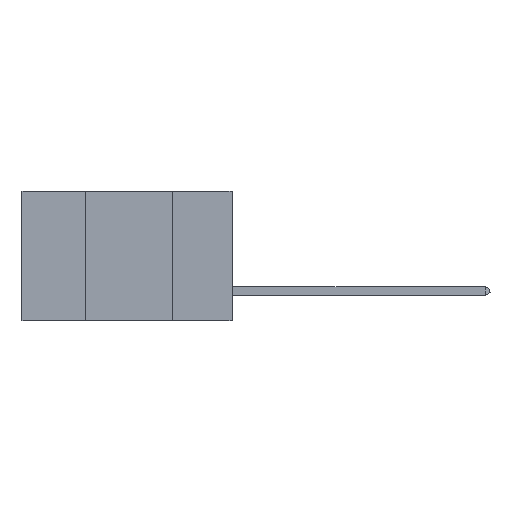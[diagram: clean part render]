
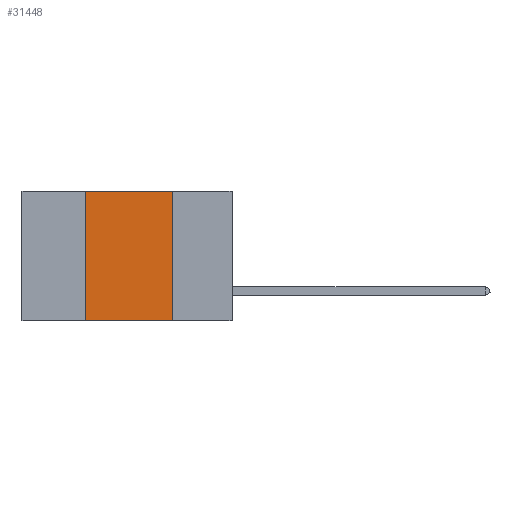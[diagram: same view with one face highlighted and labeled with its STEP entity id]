
A CAD part, left-side view. The second image highlights one B-rep face of the part: STEP entity #31448.
In plain terms, the highlighted planar face has unit normal (-1, 0, 0).
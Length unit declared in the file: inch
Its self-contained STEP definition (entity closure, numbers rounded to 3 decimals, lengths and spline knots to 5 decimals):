
#266 = DIRECTION ( 'NONE',  ( 0., 0., -1. ) ) ;
#690 = ORIENTED_EDGE ( 'NONE', *, *, #11019, .F. ) ;
#1358 = VECTOR ( 'NONE', #37948, 39.37008 ) ;
#2021 = EDGE_CURVE ( 'NONE', #32780, #37508, #21217, .T. ) ;
#4094 = DIRECTION ( 'NONE',  ( 0., 0., 1. ) ) ;
#4104 = CARTESIAN_POINT ( 'NONE',  ( 0., 0.17, -0.37 ) ) ;
#5869 = EDGE_CURVE ( 'NONE', #28290, #11673, #15813, .T. ) ;
#7186 = VECTOR ( 'NONE', #20740, 39.37008 ) ;
#7643 = VECTOR ( 'NONE', #4094, 39.37008 ) ;
#8463 = LINE ( 'NONE', #36916, #17002 ) ;
#8786 = AXIS2_PLACEMENT_3D ( 'NONE', #42294, #29114, #266 ) ;
#10260 = PLANE ( 'NONE',  #8786 ) ;
#10700 = ORIENTED_EDGE ( 'NONE', *, *, #42825, .F. ) ;
#11019 = EDGE_CURVE ( 'NONE', #11673, #37508, #8463, .T. ) ;
#11673 = VERTEX_POINT ( 'NONE', #22705 ) ;
#15813 = LINE ( 'NONE', #23886, #7186 ) ;
#16842 = EDGE_LOOP ( 'NONE', ( #690, #37872, #10700, #44517 ) ) ;
#17002 = VECTOR ( 'NONE', #44181, 39.37008 ) ;
#20740 = DIRECTION ( 'NONE',  ( 0., -1., 0. ) ) ;
#21217 = LINE ( 'NONE', #30067, #1358 ) ;
#22705 = CARTESIAN_POINT ( 'NONE',  ( 0., 0.17, 0. ) ) ;
#23886 = CARTESIAN_POINT ( 'NONE',  ( 0., 0.6, 0. ) ) ;
#24472 = CARTESIAN_POINT ( 'NONE',  ( 0., 0.42, 0. ) ) ;
#28290 = VERTEX_POINT ( 'NONE', #24472 ) ;
#29114 = DIRECTION ( 'NONE',  ( 1., 0., 0. ) ) ;
#29295 = FACE_OUTER_BOUND ( 'NONE', #16842, .T. ) ;
#29753 = LINE ( 'NONE', #44029, #7643 ) ;
#30067 = CARTESIAN_POINT ( 'NONE',  ( 0., 0.6, -0.37 ) ) ;
#31448 = ADVANCED_FACE ( 'NONE', ( #29295 ), #10260, .F. ) ;
#32780 = VERTEX_POINT ( 'NONE', #36390 ) ;
#36390 = CARTESIAN_POINT ( 'NONE',  ( 0., 0.42, -0.37 ) ) ;
#36916 = CARTESIAN_POINT ( 'NONE',  ( 0., 0.17, 0. ) ) ;
#37508 = VERTEX_POINT ( 'NONE', #4104 ) ;
#37872 = ORIENTED_EDGE ( 'NONE', *, *, #5869, .F. ) ;
#37948 = DIRECTION ( 'NONE',  ( 0., -1., 0. ) ) ;
#42294 = CARTESIAN_POINT ( 'NONE',  ( 0., 0.6, 0. ) ) ;
#42825 = EDGE_CURVE ( 'NONE', #32780, #28290, #29753, .T. ) ;
#44029 = CARTESIAN_POINT ( 'NONE',  ( 0., 0.42, 0. ) ) ;
#44181 = DIRECTION ( 'NONE',  ( 0., 0., -1. ) ) ;
#44517 = ORIENTED_EDGE ( 'NONE', *, *, #2021, .T. ) ;
